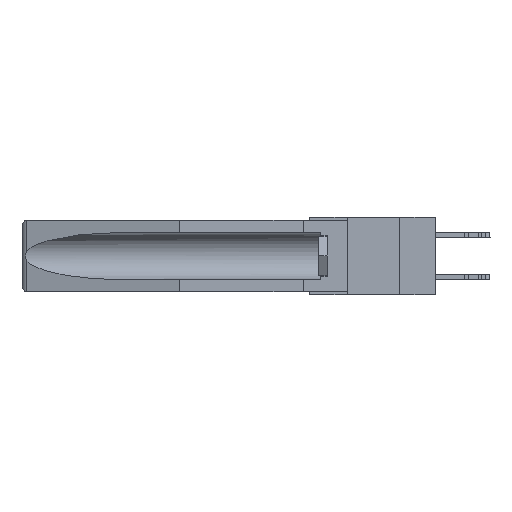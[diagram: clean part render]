
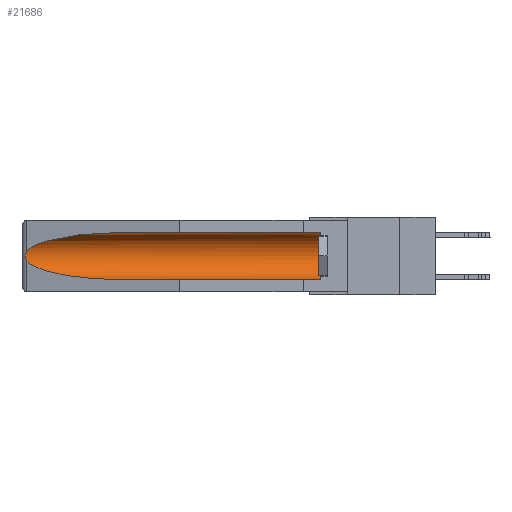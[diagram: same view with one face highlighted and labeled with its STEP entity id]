
A CAD part, left-side view. The second image highlights one B-rep face of the part: STEP entity #21686.
In plain terms, the highlighted cylindrical face has radius 2.857 mm (diameter 5.715 mm), a partial arc.
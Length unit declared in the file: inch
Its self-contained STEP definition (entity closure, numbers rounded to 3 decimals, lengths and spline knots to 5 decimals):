
#1104 = CARTESIAN_POINT ( 'NONE',  ( 0.26537, 1.52718, -0.19328 ) ) ;
#1305 = CARTESIAN_POINT ( 'NONE',  ( 0.155, 0.126, -0.284 ) ) ;
#2376 = CARTESIAN_POINT ( 'NONE',  ( 0.26537, 1.52718, -0.19328 ) ) ;
#2697 = B_SPLINE_CURVE_WITH_KNOTS ( 'NONE', 3,
 ( #19941, #7650, #25167, #4773, #22350, #9925, #10149, #27784, #27676, #25278 ),
 .UNSPECIFIED., .F., .F.,
 ( 4, 2, 2, 2, 4 ),
 ( 0., 0.00029, 0.00058, 0.00087, 0.00117 ),
 .UNSPECIFIED. ) ;
#2803 = EDGE_CURVE ( 'NONE', #16987, #13695, #16575, .T. ) ;
#3167 = DIRECTION ( 'NONE',  ( 0., 0., 1. ) ) ;
#3695 = DIRECTION ( 'NONE',  ( 0., 0., 1. ) ) ;
#4071 = CARTESIAN_POINT ( 'NONE',  ( 0.21114, 1.30732, -0.284 ) ) ;
#4773 = CARTESIAN_POINT ( 'NONE',  ( 0.2673, 1.5327, -0.16383 ) ) ;
#6008 = EDGE_CURVE ( 'NONE', #30940, #16421, #11099, .T. ) ;
#6478 = EDGE_CURVE ( 'NONE', #13695, #15750, #13918, .T. ) ;
#7472 = CARTESIAN_POINT ( 'NONE',  ( 0.155, 1.07973, -0.059 ) ) ;
#7650 = CARTESIAN_POINT ( 'NONE',  ( 0.26597, 1.52961, -0.15275 ) ) ;
#8320 = ORIENTED_EDGE ( 'NONE', *, *, #6478, .T. ) ;
#9140 = ORIENTED_EDGE ( 'NONE', *, *, #2803, .T. ) ;
#9925 = CARTESIAN_POINT ( 'NONE',  ( 0.2675, 1.53308, -0.17534 ) ) ;
#10091 = DIRECTION ( 'NONE',  ( 0., 1., 0. ) ) ;
#10149 = CARTESIAN_POINT ( 'NONE',  ( 0.2673, 1.53269, -0.17917 ) ) ;
#10821 = ORIENTED_EDGE ( 'NONE', *, *, #24553, .T. ) ;
#10845 = AXIS2_PLACEMENT_3D ( 'NONE', #15679, #23686, #3167 ) ;
#11099 = LINE ( 'NONE', #18002, #13425 ) ;
#11319 = ORIENTED_EDGE ( 'NONE', *, *, #22525, .T. ) ;
#11392 = DIRECTION ( 'NONE',  ( 0., 1., 0. ) ) ;
#11473 = FACE_OUTER_BOUND ( 'NONE', #17878, .T. ) ;
#13425 = VECTOR ( 'NONE', #10091, 39.37008 ) ;
#13695 = VERTEX_POINT ( 'NONE', #28085 ) ;
#13816 = VECTOR ( 'NONE', #18619, 39.37008 ) ;
#13918 =( BOUNDED_CURVE ( )  B_SPLINE_CURVE ( 3, ( #7472, #19869, #22390, #32198 ),
 .UNSPECIFIED., .F., .F. ) 
 B_SPLINE_CURVE_WITH_KNOTS ( ( 4, 4 ),
 ( 4.71239, 6.08839 ),
 .UNSPECIFIED. ) 
 CURVE ( )  GEOMETRIC_REPRESENTATION_ITEM ( )  RATIONAL_B_SPLINE_CURVE ( ( 1., 0.848, 0.848, 1. ) ) 
 REPRESENTATION_ITEM ( '' )  );
#15386 = CARTESIAN_POINT ( 'NONE',  ( 0.155, -0.30754, -0.059 ) ) ;
#15679 = CARTESIAN_POINT ( 'NONE',  ( 0.155, 0.126, -0.1715 ) ) ;
#15750 = VERTEX_POINT ( 'NONE', #22410 ) ;
#16421 = VERTEX_POINT ( 'NONE', #20343 ) ;
#16575 = LINE ( 'NONE', #15386, #13816 ) ;
#16987 = VERTEX_POINT ( 'NONE', #22661 ) ;
#17878 = EDGE_LOOP ( 'NONE', ( #8320, #11319, #10821, #30079, #24750, #9140 ) ) ;
#18002 = CARTESIAN_POINT ( 'NONE',  ( 0.155, -0.30754, -0.284 ) ) ;
#18619 = DIRECTION ( 'NONE',  ( 0., 1., 0. ) ) ;
#19869 = CARTESIAN_POINT ( 'NONE',  ( 0.21114, 1.30732, -0.059 ) ) ;
#19941 = CARTESIAN_POINT ( 'NONE',  ( 0.26537, 1.52718, -0.14972 ) ) ;
#20127 = CYLINDRICAL_SURFACE ( 'NONE', #20930, 0.1125 ) ;
#20343 = CARTESIAN_POINT ( 'NONE',  ( 0.155, 1.07973, -0.284 ) ) ;
#20930 = AXIS2_PLACEMENT_3D ( 'NONE', #29106, #11392, #3695 ) ;
#21541 = EDGE_CURVE ( 'NONE', #30940, #16987, #26777, .T. ) ;
#21686 = ADVANCED_FACE ( 'NONE', ( #11473 ), #20127, .F. ) ;
#22350 = CARTESIAN_POINT ( 'NONE',  ( 0.2675, 1.53308, -0.16763 ) ) ;
#22390 = CARTESIAN_POINT ( 'NONE',  ( 0.25451, 1.48313, -0.09465 ) ) ;
#22410 = CARTESIAN_POINT ( 'NONE',  ( 0.26537, 1.52718, -0.14972 ) ) ;
#22525 = EDGE_CURVE ( 'NONE', #15750, #25073, #2697, .T. ) ;
#22661 = CARTESIAN_POINT ( 'NONE',  ( 0.155, 0.126, -0.059 ) ) ;
#23686 = DIRECTION ( 'NONE',  ( 0., -1., 0. ) ) ;
#24553 = EDGE_CURVE ( 'NONE', #25073, #16421, #28981, .T. ) ;
#24750 = ORIENTED_EDGE ( 'NONE', *, *, #21541, .T. ) ;
#25073 = VERTEX_POINT ( 'NONE', #2376 ) ;
#25167 = CARTESIAN_POINT ( 'NONE',  ( 0.26654, 1.53092, -0.15636 ) ) ;
#25278 = CARTESIAN_POINT ( 'NONE',  ( 0.26537, 1.52718, -0.19328 ) ) ;
#26777 = CIRCLE ( 'NONE', #10845, 0.1125 ) ;
#27676 = CARTESIAN_POINT ( 'NONE',  ( 0.26597, 1.5296, -0.19026 ) ) ;
#27784 = CARTESIAN_POINT ( 'NONE',  ( 0.26655, 1.53094, -0.18657 ) ) ;
#28085 = CARTESIAN_POINT ( 'NONE',  ( 0.155, 1.07973, -0.059 ) ) ;
#28726 = CARTESIAN_POINT ( 'NONE',  ( 0.25451, 1.48313, -0.24835 ) ) ;
#28981 =( BOUNDED_CURVE ( )  B_SPLINE_CURVE ( 3, ( #1104, #28726, #4071, #32018 ),
 .UNSPECIFIED., .F., .T. ) 
 B_SPLINE_CURVE_WITH_KNOTS ( ( 4, 4 ),
 ( 0.1948, 1.5708 ),
 .UNSPECIFIED. ) 
 CURVE ( )  GEOMETRIC_REPRESENTATION_ITEM ( )  RATIONAL_B_SPLINE_CURVE ( ( 1., 0.848, 0.848, 1. ) ) 
 REPRESENTATION_ITEM ( '' )  );
#29106 = CARTESIAN_POINT ( 'NONE',  ( 0.155, -0.30754, -0.1715 ) ) ;
#30079 = ORIENTED_EDGE ( 'NONE', *, *, #6008, .F. ) ;
#30940 = VERTEX_POINT ( 'NONE', #1305 ) ;
#32018 = CARTESIAN_POINT ( 'NONE',  ( 0.155, 1.07973, -0.284 ) ) ;
#32198 = CARTESIAN_POINT ( 'NONE',  ( 0.26537, 1.52718, -0.14972 ) ) ;
